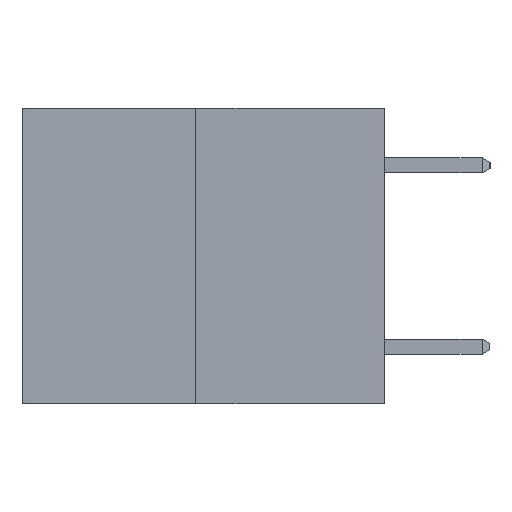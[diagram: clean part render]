
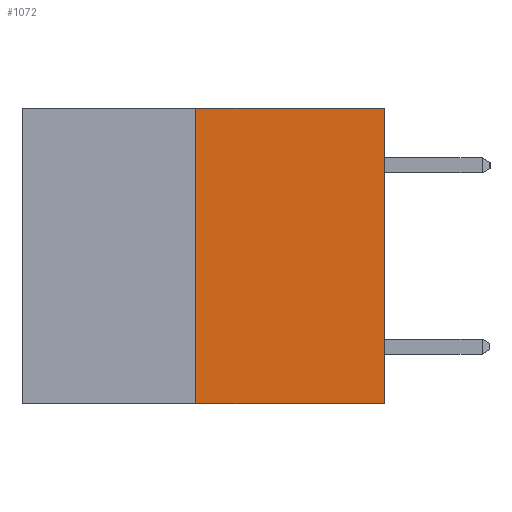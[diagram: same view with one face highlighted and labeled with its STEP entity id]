
A CAD part, left-side view. The second image highlights one B-rep face of the part: STEP entity #1072.
In plain terms, the highlighted planar face has unit normal (-1, 0, 0).
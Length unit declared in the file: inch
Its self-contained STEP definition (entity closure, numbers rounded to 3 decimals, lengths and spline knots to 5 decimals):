
#161 = CARTESIAN_POINT ( 'NONE',  ( 0., 0.312, 0. ) ) ;
#673 = VERTEX_POINT ( 'NONE', #9874 ) ;
#1071 = CARTESIAN_POINT ( 'NONE',  ( 0., 0., 0. ) ) ;
#1072 = ADVANCED_FACE ( 'NONE', ( #13540 ), #8739, .F. ) ;
#1149 = AXIS2_PLACEMENT_3D ( 'NONE', #2615, #2712, #12402 ) ;
#1291 = CARTESIAN_POINT ( 'NONE',  ( 0., 0.6, -0.49 ) ) ;
#2033 = EDGE_CURVE ( 'NONE', #5073, #5670, #8576, .T. ) ;
#2194 = EDGE_CURVE ( 'NONE', #673, #5073, #13732, .T. ) ;
#2615 = CARTESIAN_POINT ( 'NONE',  ( 0., 0.6, 0. ) ) ;
#2712 = DIRECTION ( 'NONE',  ( 1., 0., 0. ) ) ;
#2895 = ORIENTED_EDGE ( 'NONE', *, *, #2033, .T. ) ;
#3295 = DIRECTION ( 'NONE',  ( 0., -1., 0. ) ) ;
#4666 = CARTESIAN_POINT ( 'NONE',  ( 0., 0.312, -0.49 ) ) ;
#4757 = EDGE_CURVE ( 'NONE', #673, #7754, #7986, .T. ) ;
#5073 = VERTEX_POINT ( 'NONE', #5633 ) ;
#5633 = CARTESIAN_POINT ( 'NONE',  ( 0., 0., -0.49 ) ) ;
#5670 = VERTEX_POINT ( 'NONE', #8382 ) ;
#5700 = VECTOR ( 'NONE', #8564, 39.37008 ) ;
#6031 = EDGE_CURVE ( 'NONE', #7754, #5670, #6262, .T. ) ;
#6262 = LINE ( 'NONE', #11279, #9608 ) ;
#6299 = ORIENTED_EDGE ( 'NONE', *, *, #6031, .F. ) ;
#6921 = DIRECTION ( 'NONE',  ( 0., 0., 1. ) ) ;
#7485 = ORIENTED_EDGE ( 'NONE', *, *, #4757, .F. ) ;
#7754 = VERTEX_POINT ( 'NONE', #161 ) ;
#7986 = LINE ( 'NONE', #4666, #13496 ) ;
#8082 = DIRECTION ( 'NONE',  ( 0., -1., 0. ) ) ;
#8382 = CARTESIAN_POINT ( 'NONE',  ( 0., 0., 0. ) ) ;
#8564 = DIRECTION ( 'NONE',  ( 0., 0., 1. ) ) ;
#8576 = LINE ( 'NONE', #1071, #5700 ) ;
#8724 = ORIENTED_EDGE ( 'NONE', *, *, #2194, .T. ) ;
#8739 = PLANE ( 'NONE',  #1149 ) ;
#9608 = VECTOR ( 'NONE', #8082, 39.37008 ) ;
#9874 = CARTESIAN_POINT ( 'NONE',  ( 0., 0.312, -0.49 ) ) ;
#11279 = CARTESIAN_POINT ( 'NONE',  ( 0., 0.6, 0. ) ) ;
#12245 = VECTOR ( 'NONE', #3295, 39.37008 ) ;
#12402 = DIRECTION ( 'NONE',  ( 0., 0., -1. ) ) ;
#12634 = EDGE_LOOP ( 'NONE', ( #7485, #8724, #2895, #6299 ) ) ;
#13496 = VECTOR ( 'NONE', #6921, 39.37008 ) ;
#13540 = FACE_OUTER_BOUND ( 'NONE', #12634, .T. ) ;
#13732 = LINE ( 'NONE', #1291, #12245 ) ;
